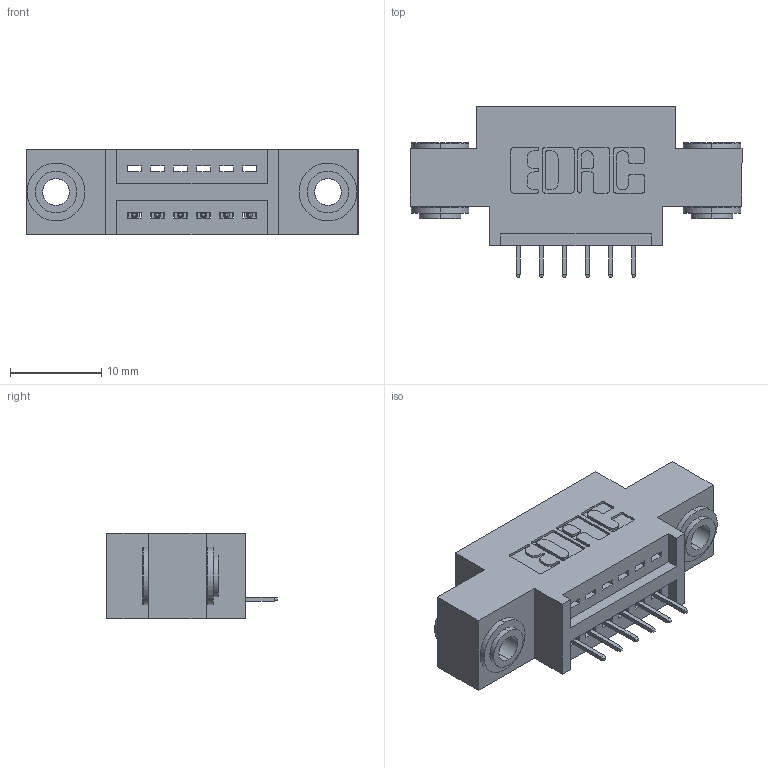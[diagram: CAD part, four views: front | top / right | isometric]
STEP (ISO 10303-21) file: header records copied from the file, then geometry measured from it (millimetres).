
FILE_DESCRIPTION (( 'STEP AP203' ), '1' );
FILE_NAME ('845-006-525-603.STEP', '2020-09-22T14:34:39', ( '' ), ( '' ), 'SwSTEP 2.0', 'SolidWorks 2020', '' );
FILE_SCHEMA (( 'CONFIG_CONTROL_DESIGN' ));
Length unit declared in the file: inch
Products named in the file (4): 845-006-525-603; 845 Part_0.170 Offset - 0.156 Dia-TH; 345-292-001_345-293-125; 345-250-002_345-250-002-102
Assembly tree (9 placements, depth 2):
  845-006-525-603
    845 Part_0.170 Offset - 0.156 Dia-TH
    345-292-001_345-293-125  x6
    345-250-002_345-250-002-102  x2
Bounding box: 36.45 x 18.72 x 9.4 mm (x, y, z)
Volume: 3048.6 mm3; surface area: 3821.3 mm2
Topology: 9 solids, 9 shells, 540 faces, 1509 edges, 978 vertices
Faces by surface type: plane 370, cylinder 162, cone 8
Entity records: 10218 total; most frequent: CARTESIAN_POINT 1749, ORIENTED_EDGE 1682, DIRECTION 1611, EDGE_CURVE 841, VECTOR 665, LINE 665, VERTEX_POINT 554, AXIS2_PLACEMENT_3D 473
